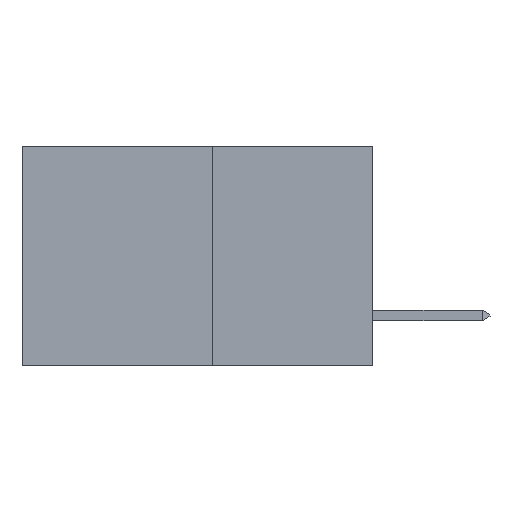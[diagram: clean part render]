
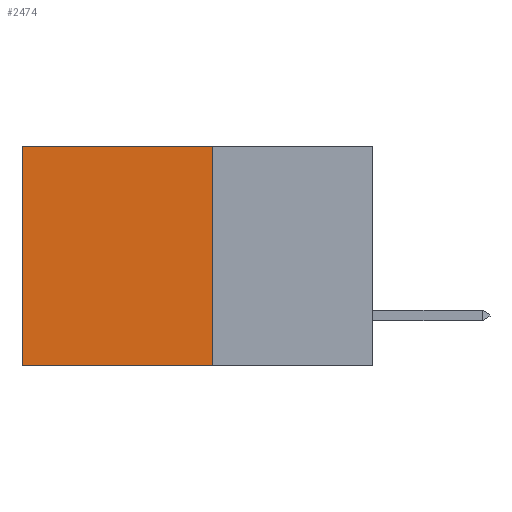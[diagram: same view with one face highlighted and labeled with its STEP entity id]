
A CAD part, left-side view. The second image highlights one B-rep face of the part: STEP entity #2474.
In plain terms, the highlighted planar face has unit normal (-1, 0, 0).
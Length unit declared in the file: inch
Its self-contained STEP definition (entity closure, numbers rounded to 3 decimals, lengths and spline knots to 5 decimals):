
#328 = CARTESIAN_POINT ( 'NONE',  ( 0.277, 0.27, -0.37 ) ) ;
#383 = ORIENTED_EDGE ( 'NONE', *, *, #11120, .T. ) ;
#394 = ORIENTED_EDGE ( 'NONE', *, *, #6961, .F. ) ;
#406 = VERTEX_POINT ( 'NONE', #8545 ) ;
#418 = ORIENTED_EDGE ( 'NONE', *, *, #1623, .F. ) ;
#428 = ORIENTED_EDGE ( 'NONE', *, *, #9711, .T. ) ;
#1623 = EDGE_CURVE ( 'NONE', #406, #9113, #8337, .T. ) ;
#1798 = VERTEX_POINT ( 'NONE', #7881 ) ;
#1881 = FACE_OUTER_BOUND ( 'NONE', #9640, .T. ) ;
#2474 = ADVANCED_FACE ( 'NONE', ( #1881 ), #10646, .F. ) ;
#2609 = CARTESIAN_POINT ( 'NONE',  ( 0.277, 0.59, -0.37 ) ) ;
#3192 = AXIS2_PLACEMENT_3D ( 'NONE', #8975, #8456, #9608 ) ;
#4819 = VERTEX_POINT ( 'NONE', #11182 ) ;
#6123 = DIRECTION ( 'NONE',  ( 0., 1., 0. ) ) ;
#6135 = VECTOR ( 'NONE', #6465, 39.37008 ) ;
#6163 = LINE ( 'NONE', #10404, #10028 ) ;
#6341 = CARTESIAN_POINT ( 'NONE',  ( 0.277, 0.27, -0.37 ) ) ;
#6465 = DIRECTION ( 'NONE',  ( 0., 0., -1. ) ) ;
#6925 = CARTESIAN_POINT ( 'NONE',  ( 0.277, 0.27, -0.37 ) ) ;
#6961 = EDGE_CURVE ( 'NONE', #9113, #4819, #8552, .T. ) ;
#7803 = VECTOR ( 'NONE', #6123, 39.37008 ) ;
#7881 = CARTESIAN_POINT ( 'NONE',  ( 0.277, 0.59, 0. ) ) ;
#8337 = LINE ( 'NONE', #328, #6135 ) ;
#8450 = VECTOR ( 'NONE', #8671, 39.37008 ) ;
#8456 = DIRECTION ( 'NONE',  ( 1., 0., 0. ) ) ;
#8545 = CARTESIAN_POINT ( 'NONE',  ( 0.277, 0.27, 0. ) ) ;
#8552 = LINE ( 'NONE', #6925, #7803 ) ;
#8671 = DIRECTION ( 'NONE',  ( 0., 0., -1. ) ) ;
#8707 = LINE ( 'NONE', #2609, #8450 ) ;
#8814 = DIRECTION ( 'NONE',  ( 0., 1., 0. ) ) ;
#8975 = CARTESIAN_POINT ( 'NONE',  ( 0.277, 0.27, -0.37 ) ) ;
#9113 = VERTEX_POINT ( 'NONE', #6341 ) ;
#9608 = DIRECTION ( 'NONE',  ( 0., 0., -1. ) ) ;
#9640 = EDGE_LOOP ( 'NONE', ( #383, #394, #418, #428 ) ) ;
#9711 = EDGE_CURVE ( 'NONE', #406, #1798, #6163, .T. ) ;
#10028 = VECTOR ( 'NONE', #8814, 39.37008 ) ;
#10404 = CARTESIAN_POINT ( 'NONE',  ( 0.277, 0.27, 0. ) ) ;
#10646 = PLANE ( 'NONE',  #3192 ) ;
#11120 = EDGE_CURVE ( 'NONE', #1798, #4819, #8707, .T. ) ;
#11182 = CARTESIAN_POINT ( 'NONE',  ( 0.277, 0.59, -0.37 ) ) ;
